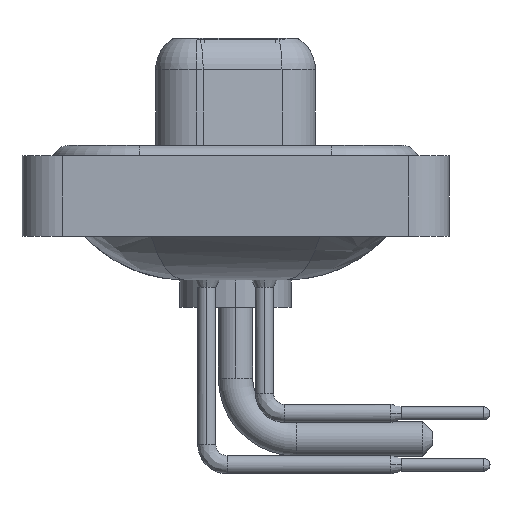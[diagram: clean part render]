
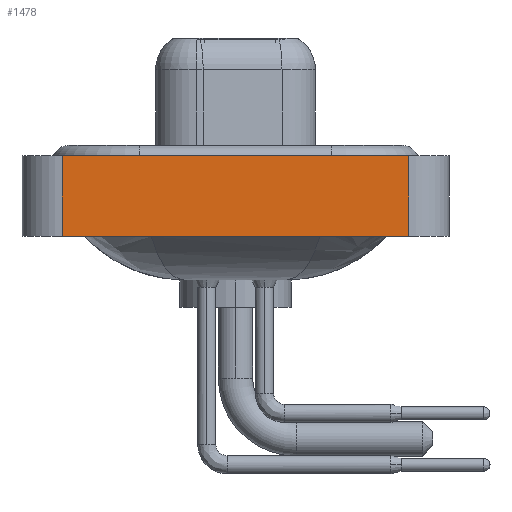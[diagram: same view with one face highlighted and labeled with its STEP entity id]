
A CAD part, left-side view. The second image highlights one B-rep face of the part: STEP entity #1478.
In plain terms, the highlighted planar face has unit normal (-1, 0, 0).
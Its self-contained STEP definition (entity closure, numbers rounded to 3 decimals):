
#13 = EDGE_CURVE ( 'NONE', #1633, #14467, #475, .T. ) ;
#381 = DIRECTION ( 'NONE',  ( 0., 0., 1. ) ) ;
#475 = LINE ( 'NONE', #6575, #11292 ) ;
#481 = ORIENTED_EDGE ( 'NONE', *, *, #23601, .T. ) ;
#906 = VECTOR ( 'NONE', #381, 1000. ) ;
#1281 = VECTOR ( 'NONE', #4931, 1000. ) ;
#1429 = EDGE_CURVE ( 'NONE', #22596, #1463, #6852, .T. ) ;
#1463 = VERTEX_POINT ( 'NONE', #13839 ) ;
#1478 = ADVANCED_FACE ( 'NONE', ( #3784 ), #19642, .T. ) ;
#1633 = VERTEX_POINT ( 'NONE', #14228 ) ;
#2493 = CARTESIAN_POINT ( 'NONE',  ( -7.35, -8.55, -3.6 ) ) ;
#2898 = EDGE_CURVE ( 'NONE', #22596, #1633, #10498, .T. ) ;
#3784 = FACE_OUTER_BOUND ( 'NONE', #22783, .T. ) ;
#3848 = CARTESIAN_POINT ( 'NONE',  ( -7.35, 8.55, -3.6 ) ) ;
#4140 = ORIENTED_EDGE ( 'NONE', *, *, #2898, .F. ) ;
#4769 = LINE ( 'NONE', #2493, #906 ) ;
#4931 = DIRECTION ( 'NONE',  ( 0., 0., 1. ) ) ;
#6575 = CARTESIAN_POINT ( 'NONE',  ( -7.35, -8.55, 0.4 ) ) ;
#6852 = LINE ( 'NONE', #23379, #7678 ) ;
#7678 = VECTOR ( 'NONE', #15087, 1000. ) ;
#8504 = CARTESIAN_POINT ( 'NONE',  ( -7.35, -8.55, 0.4 ) ) ;
#10498 = LINE ( 'NONE', #21551, #1281 ) ;
#11292 = VECTOR ( 'NONE', #20825, 1000. ) ;
#13839 = CARTESIAN_POINT ( 'NONE',  ( -7.35, -8.55, -3.6 ) ) ;
#14228 = CARTESIAN_POINT ( 'NONE',  ( -7.35, 8.55, 0.4 ) ) ;
#14467 = VERTEX_POINT ( 'NONE', #8504 ) ;
#14951 = ORIENTED_EDGE ( 'NONE', *, *, #13, .F. ) ;
#15087 = DIRECTION ( 'NONE',  ( 0., -1., 0. ) ) ;
#17596 = DIRECTION ( 'NONE',  ( 0., 0., 1. ) ) ;
#17981 = DIRECTION ( 'NONE',  ( -1., 0., 0. ) ) ;
#18318 = AXIS2_PLACEMENT_3D ( 'NONE', #21868, #17981, #17596 ) ;
#19635 = ORIENTED_EDGE ( 'NONE', *, *, #1429, .T. ) ;
#19642 = PLANE ( 'NONE',  #18318 ) ;
#20825 = DIRECTION ( 'NONE',  ( 0., -1., 0. ) ) ;
#21551 = CARTESIAN_POINT ( 'NONE',  ( -7.35, 8.55, -3.6 ) ) ;
#21868 = CARTESIAN_POINT ( 'NONE',  ( -7.35, -8.55, -3.6 ) ) ;
#22596 = VERTEX_POINT ( 'NONE', #3848 ) ;
#22783 = EDGE_LOOP ( 'NONE', ( #481, #14951, #4140, #19635 ) ) ;
#23379 = CARTESIAN_POINT ( 'NONE',  ( -7.35, -8.55, -3.6 ) ) ;
#23601 = EDGE_CURVE ( 'NONE', #1463, #14467, #4769, .T. ) ;
